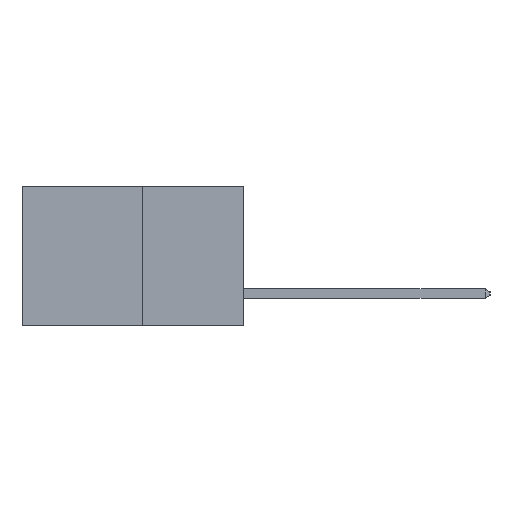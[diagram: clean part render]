
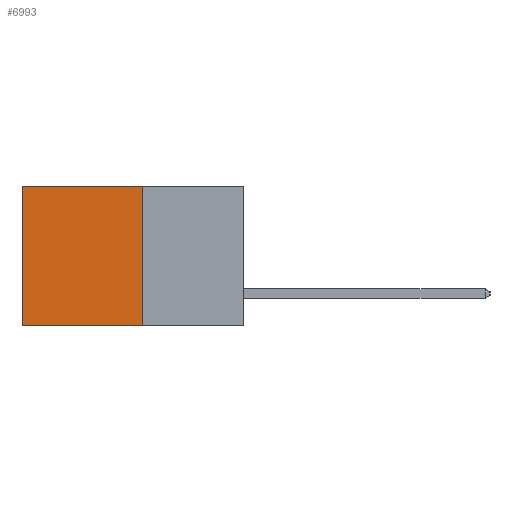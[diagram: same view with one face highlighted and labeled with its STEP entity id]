
A CAD part, left-side view. The second image highlights one B-rep face of the part: STEP entity #6993.
In plain terms, the highlighted planar face has unit normal (-1, 0, 0).
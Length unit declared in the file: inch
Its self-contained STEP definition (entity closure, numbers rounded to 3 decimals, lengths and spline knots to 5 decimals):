
#198 = LINE ( 'NONE', #2140, #6169 ) ;
#330 = EDGE_CURVE ( 'NONE', #7721, #2871, #2675, .T. ) ;
#1206 = CARTESIAN_POINT ( 'NONE',  ( 0.277, 0.27, -0.37 ) ) ;
#2140 = CARTESIAN_POINT ( 'NONE',  ( 0.277, 0.27, -0.37 ) ) ;
#2595 = VECTOR ( 'NONE', #5792, 39.37008 ) ;
#2675 = LINE ( 'NONE', #7333, #7765 ) ;
#2861 = CARTESIAN_POINT ( 'NONE',  ( 0.277, 0.27, 0. ) ) ;
#2871 = VERTEX_POINT ( 'NONE', #1206 ) ;
#3340 = VERTEX_POINT ( 'NONE', #8786 ) ;
#4100 = PLANE ( 'NONE',  #11898 ) ;
#4638 = EDGE_CURVE ( 'NONE', #9130, #3340, #11037, .T. ) ;
#5641 = ORIENTED_EDGE ( 'NONE', *, *, #7298, .F. ) ;
#5707 = FACE_OUTER_BOUND ( 'NONE', #8248, .T. ) ;
#5792 = DIRECTION ( 'NONE',  ( 0., 1., 0. ) ) ;
#6070 = DIRECTION ( 'NONE',  ( 0., 0., -1. ) ) ;
#6169 = VECTOR ( 'NONE', #8319, 39.37008 ) ;
#6993 = ADVANCED_FACE ( 'NONE', ( #5707 ), #4100, .F. ) ;
#7298 = EDGE_CURVE ( 'NONE', #2871, #3340, #198, .T. ) ;
#7333 = CARTESIAN_POINT ( 'NONE',  ( 0.277, 0.27, -0.37 ) ) ;
#7721 = VERTEX_POINT ( 'NONE', #2861 ) ;
#7765 = VECTOR ( 'NONE', #10185, 39.37008 ) ;
#8187 = DIRECTION ( 'NONE',  ( 0., 0., -1. ) ) ;
#8241 = ORIENTED_EDGE ( 'NONE', *, *, #330, .F. ) ;
#8248 = EDGE_LOOP ( 'NONE', ( #10470, #5641, #8241, #10778 ) ) ;
#8319 = DIRECTION ( 'NONE',  ( 0., 1., 0. ) ) ;
#8786 = CARTESIAN_POINT ( 'NONE',  ( 0.277, 0.59, -0.37 ) ) ;
#9130 = VERTEX_POINT ( 'NONE', #13069 ) ;
#10185 = DIRECTION ( 'NONE',  ( 0., 0., -1. ) ) ;
#10470 = ORIENTED_EDGE ( 'NONE', *, *, #4638, .T. ) ;
#10729 = VECTOR ( 'NONE', #8187, 39.37008 ) ;
#10778 = ORIENTED_EDGE ( 'NONE', *, *, #10902, .T. ) ;
#10873 = CARTESIAN_POINT ( 'NONE',  ( 0.277, 0.27, -0.37 ) ) ;
#10902 = EDGE_CURVE ( 'NONE', #7721, #9130, #12775, .T. ) ;
#11037 = LINE ( 'NONE', #11968, #10729 ) ;
#11528 = CARTESIAN_POINT ( 'NONE',  ( 0.277, 0.27, 0. ) ) ;
#11801 = DIRECTION ( 'NONE',  ( 1., 0., 0. ) ) ;
#11898 = AXIS2_PLACEMENT_3D ( 'NONE', #10873, #11801, #6070 ) ;
#11968 = CARTESIAN_POINT ( 'NONE',  ( 0.277, 0.59, -0.37 ) ) ;
#12775 = LINE ( 'NONE', #11528, #2595 ) ;
#13069 = CARTESIAN_POINT ( 'NONE',  ( 0.277, 0.59, 0. ) ) ;
